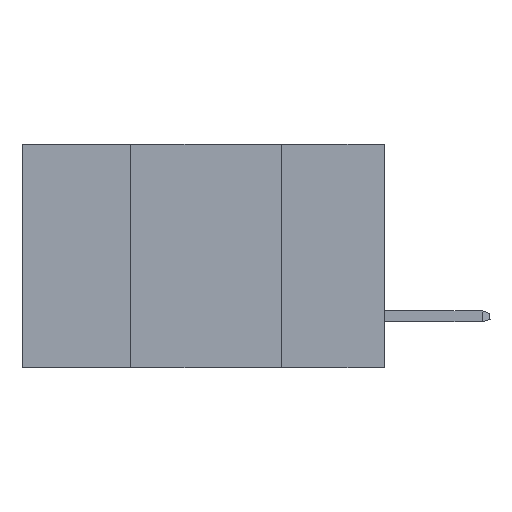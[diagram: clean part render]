
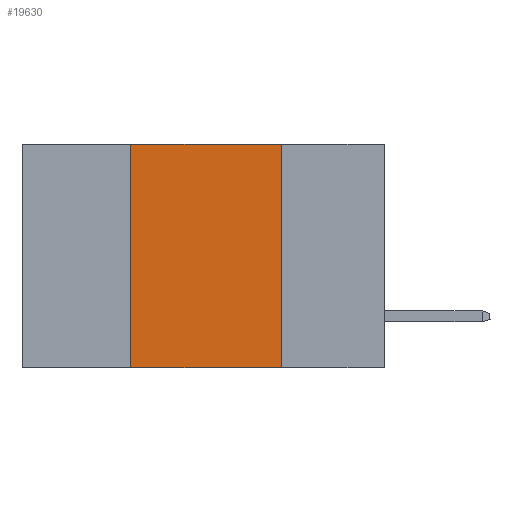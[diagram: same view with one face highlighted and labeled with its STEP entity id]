
A CAD part, left-side view. The second image highlights one B-rep face of the part: STEP entity #19630.
In plain terms, the highlighted planar face has unit normal (-1, 0, 0).
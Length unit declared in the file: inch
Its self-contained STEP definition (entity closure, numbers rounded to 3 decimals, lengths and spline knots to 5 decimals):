
#399 = EDGE_LOOP ( 'NONE', ( #8594, #20901, #19868, #10410 ) ) ;
#796 = CARTESIAN_POINT ( 'NONE',  ( 0., 0.42, 0. ) ) ;
#1775 = CARTESIAN_POINT ( 'NONE',  ( 0., 0.17, -0.37 ) ) ;
#4694 = DIRECTION ( 'NONE',  ( 0., -1., 0. ) ) ;
#4795 = LINE ( 'NONE', #13540, #22208 ) ;
#5056 = VERTEX_POINT ( 'NONE', #1775 ) ;
#5286 = VERTEX_POINT ( 'NONE', #796 ) ;
#5793 = FACE_OUTER_BOUND ( 'NONE', #399, .T. ) ;
#6057 = DIRECTION ( 'NONE',  ( 0., -1., 0. ) ) ;
#7236 = LINE ( 'NONE', #20295, #17165 ) ;
#8292 = CARTESIAN_POINT ( 'NONE',  ( 0., 0.6, 0. ) ) ;
#8594 = ORIENTED_EDGE ( 'NONE', *, *, #19000, .F. ) ;
#9395 = CARTESIAN_POINT ( 'NONE',  ( 0., 0.17, 0. ) ) ;
#9881 = LINE ( 'NONE', #9395, #22577 ) ;
#10058 = DIRECTION ( 'NONE',  ( 0., 0., -1. ) ) ;
#10410 = ORIENTED_EDGE ( 'NONE', *, *, #20199, .T. ) ;
#11707 = VERTEX_POINT ( 'NONE', #20775 ) ;
#11973 = VERTEX_POINT ( 'NONE', #14603 ) ;
#12151 = LINE ( 'NONE', #19339, #19039 ) ;
#13540 = CARTESIAN_POINT ( 'NONE',  ( 0., 0.42, 0. ) ) ;
#13610 = DIRECTION ( 'NONE',  ( 0., 0., 1. ) ) ;
#14603 = CARTESIAN_POINT ( 'NONE',  ( 0., 0.17, 0. ) ) ;
#16520 = EDGE_CURVE ( 'NONE', #11707, #5286, #4795, .T. ) ;
#17165 = VECTOR ( 'NONE', #4694, 39.37008 ) ;
#17375 = PLANE ( 'NONE',  #21294 ) ;
#17712 = EDGE_CURVE ( 'NONE', #5286, #11973, #12151, .T. ) ;
#18244 = DIRECTION ( 'NONE',  ( 0., 0., -1. ) ) ;
#19000 = EDGE_CURVE ( 'NONE', #11973, #5056, #9881, .T. ) ;
#19039 = VECTOR ( 'NONE', #6057, 39.37008 ) ;
#19339 = CARTESIAN_POINT ( 'NONE',  ( 0., 0.6, 0. ) ) ;
#19630 = ADVANCED_FACE ( 'NONE', ( #5793 ), #17375, .F. ) ;
#19868 = ORIENTED_EDGE ( 'NONE', *, *, #16520, .F. ) ;
#20199 = EDGE_CURVE ( 'NONE', #11707, #5056, #7236, .T. ) ;
#20295 = CARTESIAN_POINT ( 'NONE',  ( 0., 0.6, -0.37 ) ) ;
#20634 = DIRECTION ( 'NONE',  ( 1., 0., 0. ) ) ;
#20775 = CARTESIAN_POINT ( 'NONE',  ( 0., 0.42, -0.37 ) ) ;
#20901 = ORIENTED_EDGE ( 'NONE', *, *, #17712, .F. ) ;
#21294 = AXIS2_PLACEMENT_3D ( 'NONE', #8292, #20634, #10058 ) ;
#22208 = VECTOR ( 'NONE', #13610, 39.37008 ) ;
#22577 = VECTOR ( 'NONE', #18244, 39.37008 ) ;
